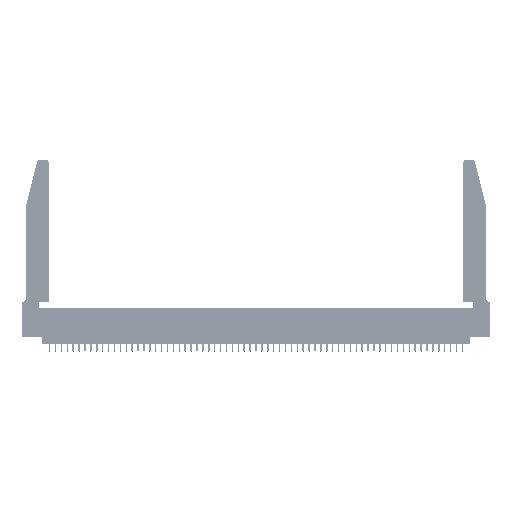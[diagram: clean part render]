
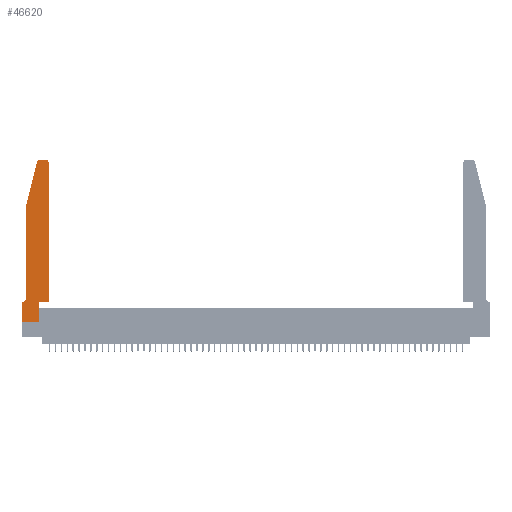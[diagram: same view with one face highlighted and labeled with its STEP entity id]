
A CAD part, top view. The second image highlights one B-rep face of the part: STEP entity #46620.
In plain terms, the highlighted planar face has unit normal (0, 0, 1).
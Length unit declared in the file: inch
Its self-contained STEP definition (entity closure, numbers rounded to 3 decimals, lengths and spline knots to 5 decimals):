
#630 = DIRECTION ( 'NONE',  ( -1., 0., 0. ) ) ;
#1775 = DIRECTION ( 'NONE',  ( 1., 0., 0. ) ) ;
#1958 = CARTESIAN_POINT ( 'NONE',  ( 0., 0., 0.37 ) ) ;
#2406 = DIRECTION ( 'NONE',  ( 1., 0., 0. ) ) ;
#3614 = DIRECTION ( 'NONE',  ( -1., 0., 0. ) ) ;
#3665 = EDGE_CURVE ( 'NONE', #25818, #30813, #39798, .T. ) ;
#5881 = CARTESIAN_POINT ( 'NONE',  ( 0., 0.35, 0.37 ) ) ;
#6323 = EDGE_CURVE ( 'NONE', #47386, #18671, #8193, .T. ) ;
#6642 = CARTESIAN_POINT ( 'NONE',  ( 0.0755, 2., 0.37 ) ) ;
#6699 = EDGE_CURVE ( 'NONE', #54261, #25818, #32708, .T. ) ;
#6886 = VERTEX_POINT ( 'NONE', #41774 ) ;
#6978 = CARTESIAN_POINT ( 'NONE',  ( 0.0055, 0.35, 0.37 ) ) ;
#7122 = CARTESIAN_POINT ( 'NONE',  ( 0.4205, 2.72, 0.37 ) ) ;
#7930 = ORIENTED_EDGE ( 'NONE', *, *, #9426, .T. ) ;
#8193 = LINE ( 'NONE', #42222, #17071 ) ;
#9332 = ORIENTED_EDGE ( 'NONE', *, *, #6699, .T. ) ;
#9409 = LINE ( 'NONE', #26539, #53135 ) ;
#9424 = VECTOR ( 'NONE', #36189, 39.37008 ) ;
#9426 = EDGE_CURVE ( 'NONE', #40810, #47386, #35914, .T. ) ;
#10334 = DIRECTION ( 'NONE',  ( 1., 0., 0. ) ) ;
#10732 = VERTEX_POINT ( 'NONE', #56009 ) ;
#10783 = ORIENTED_EDGE ( 'NONE', *, *, #51870, .T. ) ;
#11367 = CIRCLE ( 'NONE', #39943, 0.03 ) ;
#11525 = DIRECTION ( 'NONE',  ( 1., 0., 0. ) ) ;
#11548 = EDGE_CURVE ( 'NONE', #25110, #35138, #9409, .T. ) ;
#12170 = EDGE_CURVE ( 'NONE', #35138, #40810, #22420, .T. ) ;
#15379 = CARTESIAN_POINT ( 'NONE',  ( 0.4505, 0.35, 0.37 ) ) ;
#15851 = ORIENTED_EDGE ( 'NONE', *, *, #6323, .T. ) ;
#16638 = ORIENTED_EDGE ( 'NONE', *, *, #11548, .T. ) ;
#16883 = CARTESIAN_POINT ( 'NONE',  ( 0.2605, 2.75, 0.37 ) ) ;
#17071 = VECTOR ( 'NONE', #38033, 39.37008 ) ;
#17902 = EDGE_CURVE ( 'NONE', #28455, #10732, #28485, .T. ) ;
#18639 = CARTESIAN_POINT ( 'NONE',  ( 0.2865, 0.35, 0.37 ) ) ;
#18671 = VERTEX_POINT ( 'NONE', #45034 ) ;
#21575 = CARTESIAN_POINT ( 'NONE',  ( 0.25487, 2.72718, 0.37 ) ) ;
#22137 = CARTESIAN_POINT ( 'NONE',  ( 0.0055, 0.42, 0.37 ) ) ;
#22420 = LINE ( 'NONE', #18639, #9424 ) ;
#22579 = CARTESIAN_POINT ( 'NONE',  ( 0.0755, 0.35, 0.37 ) ) ;
#23053 = AXIS2_PLACEMENT_3D ( 'NONE', #22137, #52660, #26518 ) ;
#23269 = CARTESIAN_POINT ( 'NONE',  ( 0.0755, 2., 0.37 ) ) ;
#24959 = LINE ( 'NONE', #1958, #46823 ) ;
#25110 = VERTEX_POINT ( 'NONE', #33001 ) ;
#25818 = VERTEX_POINT ( 'NONE', #6642 ) ;
#26215 = ORIENTED_EDGE ( 'NONE', *, *, #48829, .T. ) ;
#26518 = DIRECTION ( 'NONE',  ( -1., 0., 0. ) ) ;
#26539 = CARTESIAN_POINT ( 'NONE',  ( 0., 0., 0.37 ) ) ;
#28094 = DIRECTION ( 'NONE',  ( 0., 0., 1. ) ) ;
#28455 = VERTEX_POINT ( 'NONE', #6978 ) ;
#28485 = LINE ( 'NONE', #22579, #38752 ) ;
#29324 = EDGE_CURVE ( 'NONE', #37634, #54261, #31924, .T. ) ;
#29612 = ORIENTED_EDGE ( 'NONE', *, *, #12170, .T. ) ;
#29749 = ORIENTED_EDGE ( 'NONE', *, *, #36038, .T. ) ;
#30100 = ORIENTED_EDGE ( 'NONE', *, *, #29324, .T. ) ;
#30783 = AXIS2_PLACEMENT_3D ( 'NONE', #54250, #28094, #1775 ) ;
#30796 = CARTESIAN_POINT ( 'NONE',  ( 0.0755, 0.42, 0.37 ) ) ;
#30813 = VERTEX_POINT ( 'NONE', #30796 ) ;
#31924 = CIRCLE ( 'NONE', #30783, 0.03 ) ;
#32074 = PLANE ( 'NONE',  #35414 ) ;
#32081 = DIRECTION ( 'NONE',  ( 0., -1., 0. ) ) ;
#32708 = LINE ( 'NONE', #23269, #34101 ) ;
#33001 = CARTESIAN_POINT ( 'NONE',  ( 0., 0., 0.37 ) ) ;
#34101 = VECTOR ( 'NONE', #53815, 39.37008 ) ;
#34558 = VECTOR ( 'NONE', #2406, 39.37008 ) ;
#35138 = VERTEX_POINT ( 'NONE', #54961 ) ;
#35414 = AXIS2_PLACEMENT_3D ( 'NONE', #5881, #36477, #10334 ) ;
#35914 = LINE ( 'NONE', #37507, #34558 ) ;
#36038 = EDGE_CURVE ( 'NONE', #6886, #37634, #50441, .T. ) ;
#36189 = DIRECTION ( 'NONE',  ( 0., 1., 0. ) ) ;
#36477 = DIRECTION ( 'NONE',  ( 0., 0., 1. ) ) ;
#37479 = VECTOR ( 'NONE', #3614, 39.37008 ) ;
#37507 = CARTESIAN_POINT ( 'NONE',  ( 0.4505, 0.35, 0.37 ) ) ;
#37634 = VERTEX_POINT ( 'NONE', #53262 ) ;
#37694 = DIRECTION ( 'NONE',  ( 0., 0., 1. ) ) ;
#38033 = DIRECTION ( 'NONE',  ( 0., 1., 0. ) ) ;
#38440 = VECTOR ( 'NONE', #55411, 39.37008 ) ;
#38752 = VECTOR ( 'NONE', #630, 39.37008 ) ;
#39798 = LINE ( 'NONE', #51032, #38440 ) ;
#39943 = AXIS2_PLACEMENT_3D ( 'NONE', #7122, #37694, #11525 ) ;
#40810 = VERTEX_POINT ( 'NONE', #43911 ) ;
#41774 = CARTESIAN_POINT ( 'NONE',  ( 0.4205, 2.75, 0.37 ) ) ;
#42222 = CARTESIAN_POINT ( 'NONE',  ( 0.4505, 0.35, 0.37 ) ) ;
#43911 = CARTESIAN_POINT ( 'NONE',  ( 0.2865, 0.35, 0.37 ) ) ;
#44476 = CIRCLE ( 'NONE', #23053, 0.07 ) ;
#44525 = EDGE_LOOP ( 'NONE', ( #29749, #30100, #9332, #45700, #26215, #44679, #10783, #16638, #29612, #7930, #15851, #55094 ) ) ;
#44679 = ORIENTED_EDGE ( 'NONE', *, *, #17902, .T. ) ;
#45034 = CARTESIAN_POINT ( 'NONE',  ( 0.4505, 2.72, 0.37 ) ) ;
#45700 = ORIENTED_EDGE ( 'NONE', *, *, #3665, .T. ) ;
#46620 = ADVANCED_FACE ( 'NONE', ( #48488 ), #32074, .T. ) ;
#46823 = VECTOR ( 'NONE', #32081, 39.37008 ) ;
#47386 = VERTEX_POINT ( 'NONE', #15379 ) ;
#48488 = FACE_OUTER_BOUND ( 'NONE', #44525, .T. ) ;
#48829 = EDGE_CURVE ( 'NONE', #30813, #28455, #44476, .T. ) ;
#50441 = LINE ( 'NONE', #16883, #37479 ) ;
#51032 = CARTESIAN_POINT ( 'NONE',  ( 0.0755, 2., 0.37 ) ) ;
#51261 = EDGE_CURVE ( 'NONE', #18671, #6886, #11367, .T. ) ;
#51870 = EDGE_CURVE ( 'NONE', #10732, #25110, #24959, .T. ) ;
#52660 = DIRECTION ( 'NONE',  ( 0., 0., -1. ) ) ;
#52684 = DIRECTION ( 'NONE',  ( 1., 0., 0. ) ) ;
#53135 = VECTOR ( 'NONE', #52684, 39.37008 ) ;
#53262 = CARTESIAN_POINT ( 'NONE',  ( 0.284, 2.75, 0.37 ) ) ;
#53815 = DIRECTION ( 'NONE',  ( -0.239, -0.971, 0. ) ) ;
#54250 = CARTESIAN_POINT ( 'NONE',  ( 0.284, 2.72, 0.37 ) ) ;
#54261 = VERTEX_POINT ( 'NONE', #21575 ) ;
#54961 = CARTESIAN_POINT ( 'NONE',  ( 0.2865, 0., 0.37 ) ) ;
#55094 = ORIENTED_EDGE ( 'NONE', *, *, #51261, .T. ) ;
#55411 = DIRECTION ( 'NONE',  ( 0., -1., 0. ) ) ;
#56009 = CARTESIAN_POINT ( 'NONE',  ( 0., 0.35, 0.37 ) ) ;
